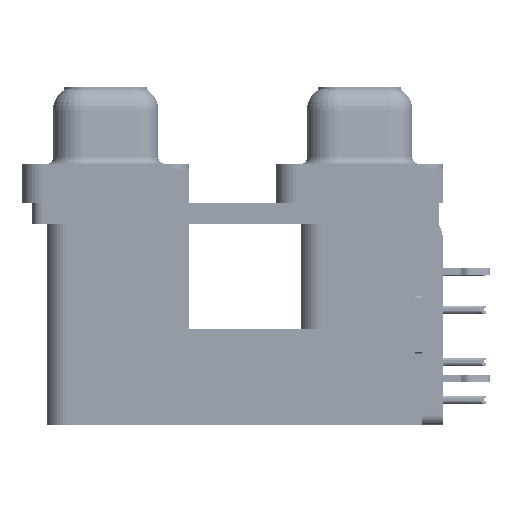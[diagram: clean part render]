
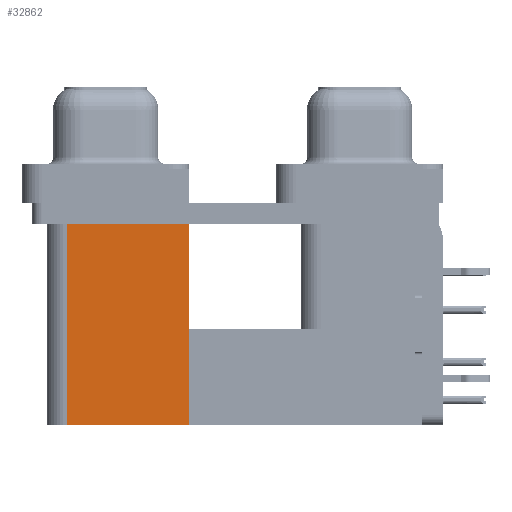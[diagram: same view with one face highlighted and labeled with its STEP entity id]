
A CAD part, left-side view. The second image highlights one B-rep face of the part: STEP entity #32862.
In plain terms, the highlighted planar face has unit normal (-1, 0, 0).
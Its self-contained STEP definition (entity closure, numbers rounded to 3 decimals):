
#1454 = DIRECTION ( 'NONE',  ( 1., 0., 0. ) ) ;
#1503 = CARTESIAN_POINT ( 'NONE',  ( 3.7, 21.975, -19.2 ) ) ;
#7131 = VECTOR ( 'NONE', #53015, 1000. ) ;
#9821 = CARTESIAN_POINT ( 'NONE',  ( 3.7, 12.775, -19.2 ) ) ;
#11086 = ORIENTED_EDGE ( 'NONE', *, *, #44097, .F. ) ;
#12421 = EDGE_LOOP ( 'NONE', ( #50232, #47562, #11086, #55179 ) ) ;
#14983 = CARTESIAN_POINT ( 'NONE',  ( 3.7, 21.975, -2.5 ) ) ;
#15384 = VECTOR ( 'NONE', #58921, 1000. ) ;
#16515 = PLANE ( 'NONE',  #34555 ) ;
#17230 = VECTOR ( 'NONE', #38060, 1000. ) ;
#18584 = EDGE_CURVE ( 'NONE', #35469, #21196, #40250, .T. ) ;
#18852 = VERTEX_POINT ( 'NONE', #1503 ) ;
#20209 = CARTESIAN_POINT ( 'NONE',  ( 3.7, 12.775, -19.2 ) ) ;
#20949 = VERTEX_POINT ( 'NONE', #45693 ) ;
#21196 = VERTEX_POINT ( 'NONE', #14983 ) ;
#31222 = LINE ( 'NONE', #36724, #55191 ) ;
#32862 = ADVANCED_FACE ( 'NONE', ( #39217 ), #16515, .F. ) ;
#34286 = EDGE_CURVE ( 'NONE', #18852, #21196, #31222, .T. ) ;
#34379 = LINE ( 'NONE', #9821, #17230 ) ;
#34555 = AXIS2_PLACEMENT_3D ( 'NONE', #20209, #1454, #43537 ) ;
#35469 = VERTEX_POINT ( 'NONE', #36773 ) ;
#36724 = CARTESIAN_POINT ( 'NONE',  ( 3.7, 21.975, -19.2 ) ) ;
#36773 = CARTESIAN_POINT ( 'NONE',  ( 3.7, 12.775, -2.5 ) ) ;
#38060 = DIRECTION ( 'NONE',  ( 0., 1., 0. ) ) ;
#39217 = FACE_OUTER_BOUND ( 'NONE', #12421, .T. ) ;
#40122 = LINE ( 'NONE', #58799, #7131 ) ;
#40250 = LINE ( 'NONE', #53754, #15384 ) ;
#43537 = DIRECTION ( 'NONE',  ( 0., 1., 0. ) ) ;
#44097 = EDGE_CURVE ( 'NONE', #20949, #18852, #34379, .T. ) ;
#45693 = CARTESIAN_POINT ( 'NONE',  ( 3.7, 12.775, -19.2 ) ) ;
#47562 = ORIENTED_EDGE ( 'NONE', *, *, #34286, .F. ) ;
#50232 = ORIENTED_EDGE ( 'NONE', *, *, #18584, .T. ) ;
#53015 = DIRECTION ( 'NONE',  ( 0., 0., 1. ) ) ;
#53754 = CARTESIAN_POINT ( 'NONE',  ( 3.7, 12.775, -2.5 ) ) ;
#55179 = ORIENTED_EDGE ( 'NONE', *, *, #58835, .T. ) ;
#55191 = VECTOR ( 'NONE', #55436, 1000. ) ;
#55436 = DIRECTION ( 'NONE',  ( 0., 0., 1. ) ) ;
#58799 = CARTESIAN_POINT ( 'NONE',  ( 3.7, 12.775, -19.2 ) ) ;
#58835 = EDGE_CURVE ( 'NONE', #20949, #35469, #40122, .T. ) ;
#58921 = DIRECTION ( 'NONE',  ( 0., 1., 0. ) ) ;
